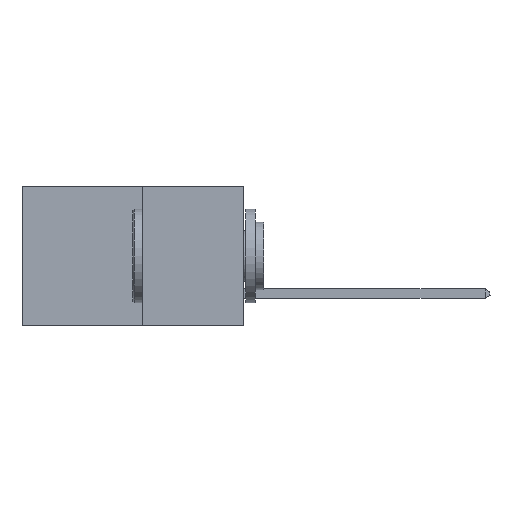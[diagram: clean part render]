
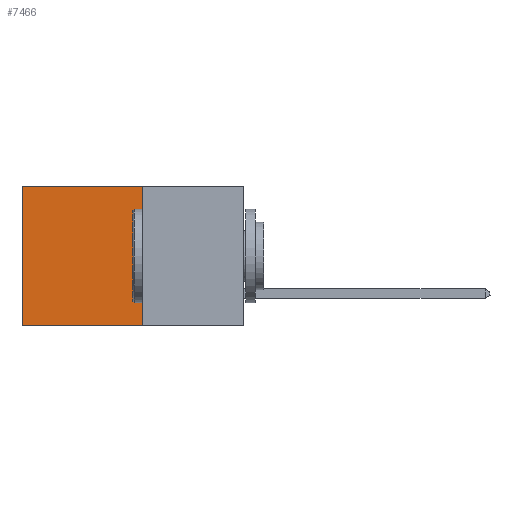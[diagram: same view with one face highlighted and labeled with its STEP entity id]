
A CAD part, left-side view. The second image highlights one B-rep face of the part: STEP entity #7466.
In plain terms, the highlighted planar face has unit normal (-1, 0, 0).
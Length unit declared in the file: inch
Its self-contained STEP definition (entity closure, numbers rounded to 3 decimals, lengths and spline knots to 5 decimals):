
#719 = CARTESIAN_POINT ( 'NONE',  ( 0.277, 0.27, 0. ) ) ;
#1041 = CARTESIAN_POINT ( 'NONE',  ( 0.277, 0.27, -0.37 ) ) ;
#1157 = EDGE_LOOP ( 'NONE', ( #10200, #10606, #12197, #11347 ) ) ;
#1223 = VECTOR ( 'NONE', #1228, 39.37008 ) ;
#1228 = DIRECTION ( 'NONE',  ( 0., 1., 0. ) ) ;
#2222 = LINE ( 'NONE', #719, #10303 ) ;
#2727 = EDGE_CURVE ( 'NONE', #9634, #12521, #2222, .T. ) ;
#3280 = VERTEX_POINT ( 'NONE', #11312 ) ;
#4088 = LINE ( 'NONE', #1041, #1223 ) ;
#4417 = DIRECTION ( 'NONE',  ( 0., 1., 0. ) ) ;
#4671 = EDGE_CURVE ( 'NONE', #12521, #3280, #11323, .T. ) ;
#5229 = CARTESIAN_POINT ( 'NONE',  ( 0.277, 0.27, -0.37 ) ) ;
#5471 = VERTEX_POINT ( 'NONE', #5229 ) ;
#6266 = CARTESIAN_POINT ( 'NONE',  ( 0.277, 0.59, 0. ) ) ;
#6312 = DIRECTION ( 'NONE',  ( 0., 0., -1. ) ) ;
#6401 = CARTESIAN_POINT ( 'NONE',  ( 0.277, 0.27, -0.37 ) ) ;
#7061 = EDGE_CURVE ( 'NONE', #9634, #5471, #11277, .T. ) ;
#7232 = EDGE_CURVE ( 'NONE', #5471, #3280, #4088, .T. ) ;
#7466 = ADVANCED_FACE ( 'NONE', ( #10945 ), #10574, .F. ) ;
#7626 = CARTESIAN_POINT ( 'NONE',  ( 0.277, 0.27, 0. ) ) ;
#8639 = VECTOR ( 'NONE', #6312, 39.37008 ) ;
#9634 = VERTEX_POINT ( 'NONE', #7626 ) ;
#10200 = ORIENTED_EDGE ( 'NONE', *, *, #4671, .T. ) ;
#10303 = VECTOR ( 'NONE', #4417, 39.37008 ) ;
#10419 = DIRECTION ( 'NONE',  ( 0., 0., -1. ) ) ;
#10461 = DIRECTION ( 'NONE',  ( 1., 0., 0. ) ) ;
#10574 = PLANE ( 'NONE',  #12654 ) ;
#10606 = ORIENTED_EDGE ( 'NONE', *, *, #7232, .F. ) ;
#10945 = FACE_OUTER_BOUND ( 'NONE', #1157, .T. ) ;
#11277 = LINE ( 'NONE', #6401, #8639 ) ;
#11312 = CARTESIAN_POINT ( 'NONE',  ( 0.277, 0.59, -0.37 ) ) ;
#11323 = LINE ( 'NONE', #12009, #13003 ) ;
#11326 = CARTESIAN_POINT ( 'NONE',  ( 0.277, 0.27, -0.37 ) ) ;
#11347 = ORIENTED_EDGE ( 'NONE', *, *, #2727, .T. ) ;
#11966 = DIRECTION ( 'NONE',  ( 0., 0., -1. ) ) ;
#12009 = CARTESIAN_POINT ( 'NONE',  ( 0.277, 0.59, -0.37 ) ) ;
#12197 = ORIENTED_EDGE ( 'NONE', *, *, #7061, .F. ) ;
#12521 = VERTEX_POINT ( 'NONE', #6266 ) ;
#12654 = AXIS2_PLACEMENT_3D ( 'NONE', #11326, #10461, #10419 ) ;
#13003 = VECTOR ( 'NONE', #11966, 39.37008 ) ;
